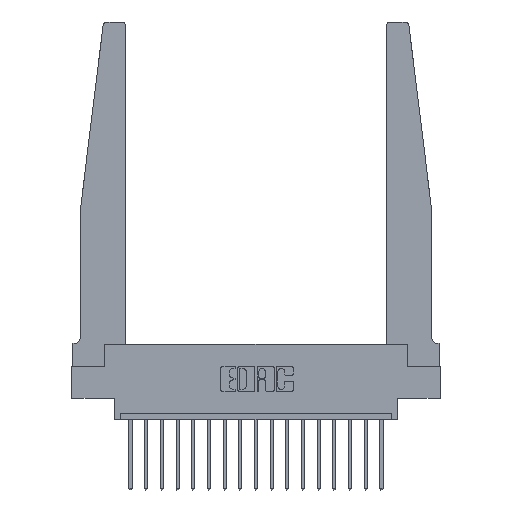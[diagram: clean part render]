
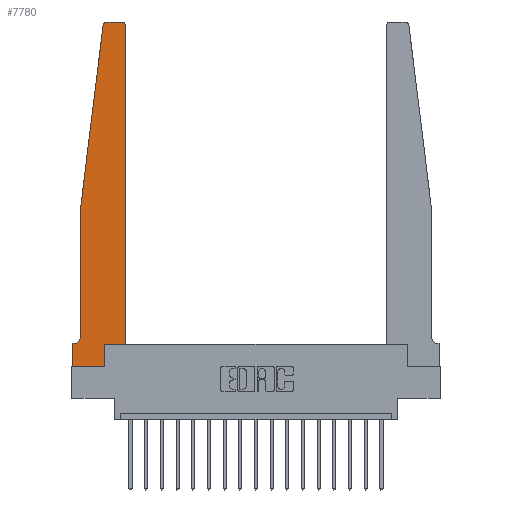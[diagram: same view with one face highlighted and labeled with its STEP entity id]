
A CAD part, top view. The second image highlights one B-rep face of the part: STEP entity #7780.
In plain terms, the highlighted planar face has unit normal (0, 0, 1).
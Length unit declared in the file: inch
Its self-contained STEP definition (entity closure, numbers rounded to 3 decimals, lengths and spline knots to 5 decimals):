
#133 = CARTESIAN_POINT ( 'NONE',  ( 0.015, 0.2375, 0.37 ) ) ;
#351 = PLANE ( 'NONE',  #13602 ) ;
#419 = CARTESIAN_POINT ( 'NONE',  ( 0.2605, 0., 0.37 ) ) ;
#424 = CARTESIAN_POINT ( 'NONE',  ( 0., 0.1875, 0.37 ) ) ;
#1216 = EDGE_CURVE ( 'NONE', #3558, #16295, #7478, .T. ) ;
#1311 = DIRECTION ( 'NONE',  ( 1., 0., 0. ) ) ;
#1404 = LINE ( 'NONE', #3954, #3308 ) ;
#2458 = CARTESIAN_POINT ( 'NONE',  ( 0.065, 0.1875, 0.37 ) ) ;
#2706 = LINE ( 'NONE', #5329, #10713 ) ;
#2790 = CARTESIAN_POINT ( 'NONE',  ( 0.27653, 2.72, 0.37 ) ) ;
#2936 = EDGE_CURVE ( 'NONE', #16295, #12458, #12033, .T. ) ;
#3176 = DIRECTION ( 'NONE',  ( 0., 0., -1. ) ) ;
#3308 = VECTOR ( 'NONE', #16127, 39.37008 ) ;
#3372 = CARTESIAN_POINT ( 'NONE',  ( 0.27653, 2.75, 0.37 ) ) ;
#3381 = CARTESIAN_POINT ( 'NONE',  ( 0., 0.1875, 0.37 ) ) ;
#3558 = VERTEX_POINT ( 'NONE', #13069 ) ;
#3592 = VECTOR ( 'NONE', #14247, 39.37008 ) ;
#3676 = VECTOR ( 'NONE', #16770, 39.37008 ) ;
#3783 = VERTEX_POINT ( 'NONE', #9624 ) ;
#3954 = CARTESIAN_POINT ( 'NONE',  ( 0.065, 1.25, 0.37 ) ) ;
#4154 = VERTEX_POINT ( 'NONE', #419 ) ;
#4259 = LINE ( 'NONE', #11677, #5095 ) ;
#4328 = CARTESIAN_POINT ( 'NONE',  ( 0.25, 2.75, 0.37 ) ) ;
#4461 = VERTEX_POINT ( 'NONE', #17384 ) ;
#5041 = VECTOR ( 'NONE', #17961, 39.37008 ) ;
#5081 = CARTESIAN_POINT ( 'NONE',  ( 0.395, 2.75, 0.37 ) ) ;
#5095 = VECTOR ( 'NONE', #10010, 39.37008 ) ;
#5329 = CARTESIAN_POINT ( 'NONE',  ( 0.065, 1.25, 0.37 ) ) ;
#5819 = VERTEX_POINT ( 'NONE', #13678 ) ;
#6110 = EDGE_CURVE ( 'NONE', #5819, #6620, #15799, .T. ) ;
#6472 = CIRCLE ( 'NONE', #8018, 0.05 ) ;
#6620 = VERTEX_POINT ( 'NONE', #424 ) ;
#6724 = ORIENTED_EDGE ( 'NONE', *, *, #6110, .T. ) ;
#6760 = VERTEX_POINT ( 'NONE', #8213 ) ;
#7163 = DIRECTION ( 'NONE',  ( -0.122, -0.992, 0. ) ) ;
#7478 = CIRCLE ( 'NONE', #18380, 0.03 ) ;
#7780 = ADVANCED_FACE ( 'NONE', ( #15177 ), #351, .T. ) ;
#8018 = AXIS2_PLACEMENT_3D ( 'NONE', #133, #3176, #17005 ) ;
#8179 = LINE ( 'NONE', #14143, #3592 ) ;
#8213 = CARTESIAN_POINT ( 'NONE',  ( 0.065, 0.2375, 0.37 ) ) ;
#8432 = ORIENTED_EDGE ( 'NONE', *, *, #17957, .T. ) ;
#8484 = DIRECTION ( 'NONE',  ( -1., 0., 0. ) ) ;
#8485 = EDGE_CURVE ( 'NONE', #6760, #5819, #6472, .T. ) ;
#8857 = ORIENTED_EDGE ( 'NONE', *, *, #16138, .T. ) ;
#9150 = LINE ( 'NONE', #15111, #3676 ) ;
#9180 = LINE ( 'NONE', #15036, #12309 ) ;
#9314 = DIRECTION ( 'NONE',  ( 0., 0., 1. ) ) ;
#9624 = CARTESIAN_POINT ( 'NONE',  ( 0.065, 1.25, 0.37 ) ) ;
#10010 = DIRECTION ( 'NONE',  ( 0., 1., 0. ) ) ;
#10597 = CARTESIAN_POINT ( 'NONE',  ( 0.2605, 0.18, 0.37 ) ) ;
#10615 = ORIENTED_EDGE ( 'NONE', *, *, #14596, .T. ) ;
#10713 = VECTOR ( 'NONE', #7163, 39.37008 ) ;
#10735 = ORIENTED_EDGE ( 'NONE', *, *, #18793, .T. ) ;
#10778 = VECTOR ( 'NONE', #8484, 39.37008 ) ;
#10781 = EDGE_CURVE ( 'NONE', #14731, #4461, #9150, .T. ) ;
#10860 = DIRECTION ( 'NONE',  ( 1., 0., 0. ) ) ;
#11677 = CARTESIAN_POINT ( 'NONE',  ( 0.425, 0.18, 0.37 ) ) ;
#11695 = ORIENTED_EDGE ( 'NONE', *, *, #2936, .T. ) ;
#11732 = ORIENTED_EDGE ( 'NONE', *, *, #15986, .T. ) ;
#12033 = LINE ( 'NONE', #4328, #5041 ) ;
#12214 = EDGE_CURVE ( 'NONE', #16094, #3783, #2706, .T. ) ;
#12309 = VECTOR ( 'NONE', #10860, 39.37008 ) ;
#12353 = AXIS2_PLACEMENT_3D ( 'NONE', #2790, #14672, #1311 ) ;
#12458 = VERTEX_POINT ( 'NONE', #3372 ) ;
#12841 = DIRECTION ( 'NONE',  ( 0., 0., 1. ) ) ;
#13023 = EDGE_LOOP ( 'NONE', ( #11695, #18859, #15656, #10735, #13104, #6724, #8432, #8857, #11732, #16949, #10615, #13398 ) ) ;
#13069 = CARTESIAN_POINT ( 'NONE',  ( 0.425, 2.72, 0.37 ) ) ;
#13104 = ORIENTED_EDGE ( 'NONE', *, *, #8485, .T. ) ;
#13398 = ORIENTED_EDGE ( 'NONE', *, *, #1216, .T. ) ;
#13602 = AXIS2_PLACEMENT_3D ( 'NONE', #3381, #9314, #18273 ) ;
#13678 = CARTESIAN_POINT ( 'NONE',  ( 0.015, 0.1875, 0.37 ) ) ;
#14143 = CARTESIAN_POINT ( 'NONE',  ( 0., 0., 0.37 ) ) ;
#14247 = DIRECTION ( 'NONE',  ( 0., -1., 0. ) ) ;
#14301 = CARTESIAN_POINT ( 'NONE',  ( 0., 0., 0.37 ) ) ;
#14498 = DIRECTION ( 'NONE',  ( 1., 0., 0. ) ) ;
#14596 = EDGE_CURVE ( 'NONE', #4461, #3558, #4259, .T. ) ;
#14672 = DIRECTION ( 'NONE',  ( 0., 0., 1. ) ) ;
#14731 = VERTEX_POINT ( 'NONE', #10597 ) ;
#14746 = LINE ( 'NONE', #16020, #17589 ) ;
#15036 = CARTESIAN_POINT ( 'NONE',  ( 0., 0., 0.37 ) ) ;
#15111 = CARTESIAN_POINT ( 'NONE',  ( 0.425, 0.18, 0.37 ) ) ;
#15177 = FACE_OUTER_BOUND ( 'NONE', #13023, .T. ) ;
#15656 = ORIENTED_EDGE ( 'NONE', *, *, #12214, .T. ) ;
#15799 = LINE ( 'NONE', #2458, #10778 ) ;
#15986 = EDGE_CURVE ( 'NONE', #4154, #14731, #14746, .T. ) ;
#16020 = CARTESIAN_POINT ( 'NONE',  ( 0.2605, 0.18, 0.37 ) ) ;
#16080 = CIRCLE ( 'NONE', #12353, 0.03 ) ;
#16094 = VERTEX_POINT ( 'NONE', #16307 ) ;
#16127 = DIRECTION ( 'NONE',  ( 0., -1., 0. ) ) ;
#16138 = EDGE_CURVE ( 'NONE', #18664, #4154, #9180, .T. ) ;
#16295 = VERTEX_POINT ( 'NONE', #5081 ) ;
#16307 = CARTESIAN_POINT ( 'NONE',  ( 0.24675, 2.72367, 0.37 ) ) ;
#16770 = DIRECTION ( 'NONE',  ( 1., 0., 0. ) ) ;
#16949 = ORIENTED_EDGE ( 'NONE', *, *, #10781, .T. ) ;
#17005 = DIRECTION ( 'NONE',  ( -1., 0., 0. ) ) ;
#17227 = CARTESIAN_POINT ( 'NONE',  ( 0.395, 2.72, 0.37 ) ) ;
#17384 = CARTESIAN_POINT ( 'NONE',  ( 0.425, 0.18, 0.37 ) ) ;
#17589 = VECTOR ( 'NONE', #19043, 39.37008 ) ;
#17957 = EDGE_CURVE ( 'NONE', #6620, #18664, #8179, .T. ) ;
#17961 = DIRECTION ( 'NONE',  ( -1., 0., 0. ) ) ;
#18273 = DIRECTION ( 'NONE',  ( 1., 0., 0. ) ) ;
#18380 = AXIS2_PLACEMENT_3D ( 'NONE', #17227, #12841, #14498 ) ;
#18664 = VERTEX_POINT ( 'NONE', #14301 ) ;
#18793 = EDGE_CURVE ( 'NONE', #3783, #6760, #1404, .T. ) ;
#18859 = ORIENTED_EDGE ( 'NONE', *, *, #18892, .T. ) ;
#18892 = EDGE_CURVE ( 'NONE', #12458, #16094, #16080, .T. ) ;
#19043 = DIRECTION ( 'NONE',  ( 0., 1., 0. ) ) ;
